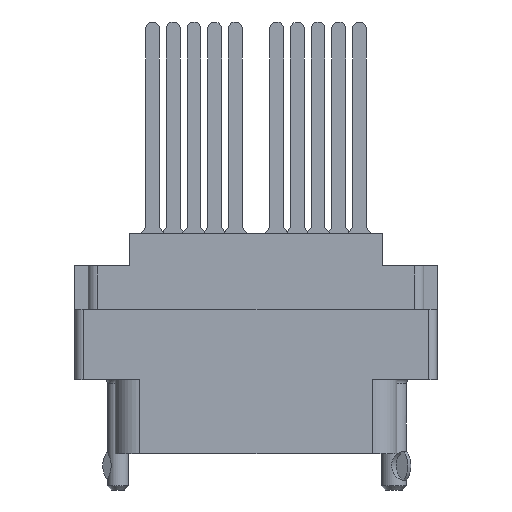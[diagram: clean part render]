
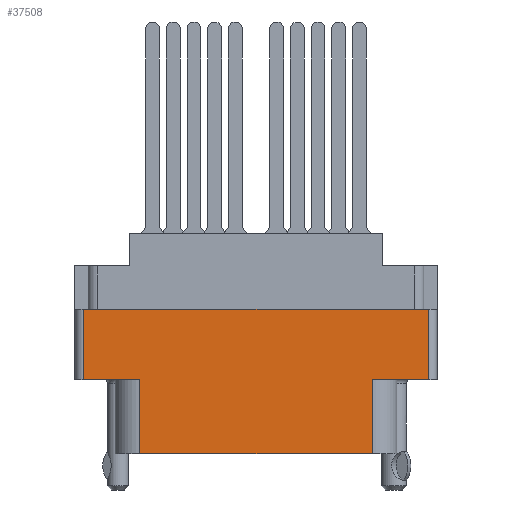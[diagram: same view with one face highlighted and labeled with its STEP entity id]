
A CAD part, front view. The second image highlights one B-rep face of the part: STEP entity #37508.
In plain terms, the highlighted planar face has unit normal (0, -1, 0).
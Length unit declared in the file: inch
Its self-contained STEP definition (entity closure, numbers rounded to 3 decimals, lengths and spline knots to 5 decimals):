
#354 = VERTEX_POINT ( 'NONE', #35522 ) ;
#2632 = CARTESIAN_POINT ( 'NONE',  ( 0.624, -0.343, -0.798 ) ) ;
#2855 = FACE_OUTER_BOUND ( 'NONE', #28072, .T. ) ;
#2922 = VERTEX_POINT ( 'NONE', #25866 ) ;
#2966 = CARTESIAN_POINT ( 'NONE',  ( -0.42052, -0.343, -0.798 ) ) ;
#3892 = CARTESIAN_POINT ( 'NONE',  ( -0.42052, -0.343, -0.529 ) ) ;
#5256 = VERTEX_POINT ( 'NONE', #37604 ) ;
#6560 = VECTOR ( 'NONE', #30645, 39.37008 ) ;
#7082 = LINE ( 'NONE', #2966, #35692 ) ;
#8413 = CARTESIAN_POINT ( 'NONE',  ( -0.624, -0.343, -0.529 ) ) ;
#9377 = LINE ( 'NONE', #33715, #36628 ) ;
#10132 = DIRECTION ( 'NONE',  ( 1., 0., 0. ) ) ;
#10142 = ORIENTED_EDGE ( 'NONE', *, *, #34833, .T. ) ;
#11123 = DIRECTION ( 'NONE',  ( 0., 0., -1. ) ) ;
#12000 = EDGE_CURVE ( 'NONE', #21095, #34467, #34928, .T. ) ;
#12207 = CARTESIAN_POINT ( 'NONE',  ( 0., -0.343, -0.529 ) ) ;
#12416 = LINE ( 'NONE', #12207, #31504 ) ;
#12677 = AXIS2_PLACEMENT_3D ( 'NONE', #15256, #29796, #18160 ) ;
#12700 = VERTEX_POINT ( 'NONE', #29169 ) ;
#13657 = VECTOR ( 'NONE', #18392, 39.37008 ) ;
#14463 = ORIENTED_EDGE ( 'NONE', *, *, #36027, .T. ) ;
#15252 = LINE ( 'NONE', #36350, #6560 ) ;
#15256 = CARTESIAN_POINT ( 'NONE',  ( -0.656, -0.343, -0.798 ) ) ;
#15358 = CARTESIAN_POINT ( 'NONE',  ( 0.42052, -0.343, -0.529 ) ) ;
#16137 = VECTOR ( 'NONE', #37226, 39.37008 ) ;
#16615 = CARTESIAN_POINT ( 'NONE',  ( 0.624, -0.343, -0.529 ) ) ;
#17618 = ORIENTED_EDGE ( 'NONE', *, *, #23342, .T. ) ;
#18160 = DIRECTION ( 'NONE',  ( 0., 0., -1. ) ) ;
#18392 = DIRECTION ( 'NONE',  ( 0., 0., 1. ) ) ;
#18929 = ORIENTED_EDGE ( 'NONE', *, *, #12000, .T. ) ;
#19539 = DIRECTION ( 'NONE',  ( 0., 0., 1. ) ) ;
#20411 = VECTOR ( 'NONE', #19539, 39.37008 ) ;
#21095 = VERTEX_POINT ( 'NONE', #16615 ) ;
#21475 = DIRECTION ( 'NONE',  ( -1., 0., 0. ) ) ;
#22395 = VERTEX_POINT ( 'NONE', #8413 ) ;
#22766 = ORIENTED_EDGE ( 'NONE', *, *, #35186, .T. ) ;
#22869 = DIRECTION ( 'NONE',  ( 0., 0., -1. ) ) ;
#23342 = EDGE_CURVE ( 'NONE', #32788, #2922, #7082, .T. ) ;
#23682 = ORIENTED_EDGE ( 'NONE', *, *, #36932, .F. ) ;
#23808 = CARTESIAN_POINT ( 'NONE',  ( 0.624, -0.343, -0.274 ) ) ;
#25244 = ORIENTED_EDGE ( 'NONE', *, *, #36755, .F. ) ;
#25866 = CARTESIAN_POINT ( 'NONE',  ( -0.42052, -0.343, -0.798 ) ) ;
#25879 = LINE ( 'NONE', #15358, #13657 ) ;
#26609 = LINE ( 'NONE', #28440, #31180 ) ;
#26940 = ORIENTED_EDGE ( 'NONE', *, *, #32630, .T. ) ;
#28072 = EDGE_LOOP ( 'NONE', ( #25244, #22766, #10142, #17618, #14463, #26940, #23682, #18929 ) ) ;
#28440 = CARTESIAN_POINT ( 'NONE',  ( -0.624, -0.343, -0.798 ) ) ;
#29169 = CARTESIAN_POINT ( 'NONE',  ( 0.42052, -0.343, -0.529 ) ) ;
#29796 = DIRECTION ( 'NONE',  ( 0., -1., 0. ) ) ;
#30645 = DIRECTION ( 'NONE',  ( 1., 0., 0. ) ) ;
#31180 = VECTOR ( 'NONE', #22869, 39.37008 ) ;
#31504 = VECTOR ( 'NONE', #21475, 39.37008 ) ;
#31544 = LINE ( 'NONE', #31649, #16137 ) ;
#31649 = CARTESIAN_POINT ( 'NONE',  ( 0., -0.343, -0.274 ) ) ;
#32630 = EDGE_CURVE ( 'NONE', #354, #12700, #25879, .T. ) ;
#32788 = VERTEX_POINT ( 'NONE', #3892 ) ;
#33119 = PLANE ( 'NONE',  #12677 ) ;
#33715 = CARTESIAN_POINT ( 'NONE',  ( 0., -0.343, -0.529 ) ) ;
#34467 = VERTEX_POINT ( 'NONE', #23808 ) ;
#34833 = EDGE_CURVE ( 'NONE', #22395, #32788, #9377, .T. ) ;
#34928 = LINE ( 'NONE', #2632, #20411 ) ;
#35186 = EDGE_CURVE ( 'NONE', #5256, #22395, #26609, .T. ) ;
#35522 = CARTESIAN_POINT ( 'NONE',  ( 0.42052, -0.343, -0.798 ) ) ;
#35692 = VECTOR ( 'NONE', #11123, 39.37008 ) ;
#36027 = EDGE_CURVE ( 'NONE', #2922, #354, #15252, .T. ) ;
#36350 = CARTESIAN_POINT ( 'NONE',  ( -0.656, -0.343, -0.798 ) ) ;
#36628 = VECTOR ( 'NONE', #10132, 39.37008 ) ;
#36755 = EDGE_CURVE ( 'NONE', #5256, #34467, #31544, .T. ) ;
#36932 = EDGE_CURVE ( 'NONE', #21095, #12700, #12416, .T. ) ;
#37226 = DIRECTION ( 'NONE',  ( 1., 0., 0. ) ) ;
#37508 = ADVANCED_FACE ( 'NONE', ( #2855 ), #33119, .T. ) ;
#37604 = CARTESIAN_POINT ( 'NONE',  ( -0.624, -0.343, -0.274 ) ) ;
